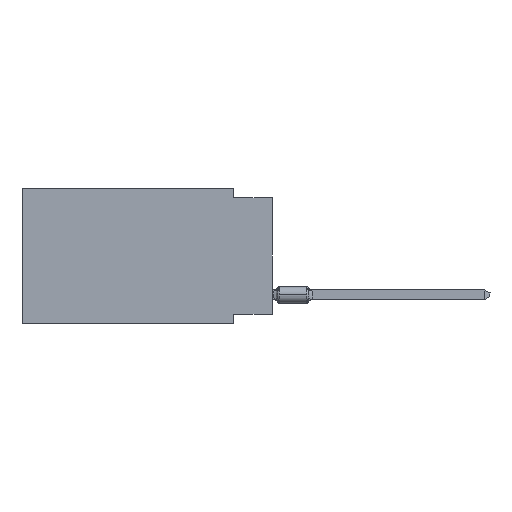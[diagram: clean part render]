
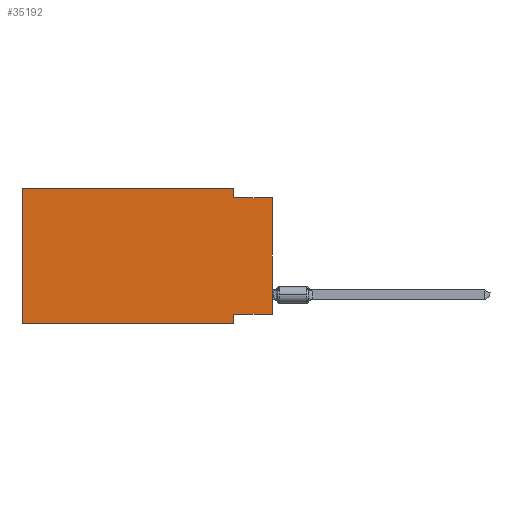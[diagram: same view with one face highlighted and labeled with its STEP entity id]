
A CAD part, left-side view. The second image highlights one B-rep face of the part: STEP entity #35192.
In plain terms, the highlighted planar face has unit normal (-1, 0, 0).
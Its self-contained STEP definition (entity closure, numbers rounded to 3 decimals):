
#883 = VECTOR ( 'NONE', #35924, 1000. ) ;
#1798 = EDGE_CURVE ( 'NONE', #45703, #31901, #57892, .T. ) ;
#2780 = VECTOR ( 'NONE', #5431, 1000. ) ;
#3551 = VECTOR ( 'NONE', #25320, 1000. ) ;
#4039 = EDGE_LOOP ( 'NONE', ( #21604, #40811, #22228, #12250, #41114, #58420, #39677, #47227 ) ) ;
#4810 = LINE ( 'NONE', #8172, #883 ) ;
#5431 = DIRECTION ( 'NONE',  ( 0., 0., 1. ) ) ;
#5694 = AXIS2_PLACEMENT_3D ( 'NONE', #21321, #26786, #53914 ) ;
#6041 = CARTESIAN_POINT ( 'NONE',  ( 0., 0., -0.635 ) ) ;
#6371 = DIRECTION ( 'NONE',  ( 0., 0., -1. ) ) ;
#7266 = CARTESIAN_POINT ( 'NONE',  ( 0., 2.54, -8.89 ) ) ;
#7728 = VECTOR ( 'NONE', #34967, 1000. ) ;
#7740 = VECTOR ( 'NONE', #36163, 1000. ) ;
#8172 = CARTESIAN_POINT ( 'NONE',  ( 0., 16.383, 0. ) ) ;
#9313 = CARTESIAN_POINT ( 'NONE',  ( 0., 2.54, -8.89 ) ) ;
#10871 = EDGE_CURVE ( 'NONE', #17451, #39127, #16458, .T. ) ;
#12250 = ORIENTED_EDGE ( 'NONE', *, *, #37661, .F. ) ;
#13617 = VECTOR ( 'NONE', #6371, 1000. ) ;
#15258 = CARTESIAN_POINT ( 'NONE',  ( 0., 16.383, 0. ) ) ;
#16373 = LINE ( 'NONE', #39853, #7728 ) ;
#16458 = LINE ( 'NONE', #15258, #3551 ) ;
#17451 = VERTEX_POINT ( 'NONE', #21964 ) ;
#17556 = CARTESIAN_POINT ( 'NONE',  ( 0., 0., -8.255 ) ) ;
#21321 = CARTESIAN_POINT ( 'NONE',  ( 0., 16.383, 0. ) ) ;
#21604 = ORIENTED_EDGE ( 'NONE', *, *, #59350, .T. ) ;
#21964 = CARTESIAN_POINT ( 'NONE',  ( 0., 16.383, -8.89 ) ) ;
#22228 = ORIENTED_EDGE ( 'NONE', *, *, #31782, .F. ) ;
#22732 = CARTESIAN_POINT ( 'NONE',  ( 0., 16.383, -8.89 ) ) ;
#25320 = DIRECTION ( 'NONE',  ( 0., 0., 1. ) ) ;
#26594 = EDGE_CURVE ( 'NONE', #46502, #45478, #47813, .T. ) ;
#26786 = DIRECTION ( 'NONE',  ( 1., 0., 0. ) ) ;
#27468 = CARTESIAN_POINT ( 'NONE',  ( 0., 2.54, -0.635 ) ) ;
#28627 = LINE ( 'NONE', #47212, #2780 ) ;
#31782 = EDGE_CURVE ( 'NONE', #58960, #46502, #16373, .T. ) ;
#31901 = VERTEX_POINT ( 'NONE', #9313 ) ;
#33528 = CARTESIAN_POINT ( 'NONE',  ( 0., 16.383, 0. ) ) ;
#34967 = DIRECTION ( 'NONE',  ( 0., 0., -1. ) ) ;
#35192 = ADVANCED_FACE ( 'NONE', ( #36250 ), #36538, .F. ) ;
#35924 = DIRECTION ( 'NONE',  ( 0., -1., 0. ) ) ;
#36163 = DIRECTION ( 'NONE',  ( 0., 1., 0. ) ) ;
#36250 = FACE_OUTER_BOUND ( 'NONE', #4039, .T. ) ;
#36538 = PLANE ( 'NONE',  #5694 ) ;
#37661 = EDGE_CURVE ( 'NONE', #39127, #58960, #4810, .T. ) ;
#39127 = VERTEX_POINT ( 'NONE', #33528 ) ;
#39677 = ORIENTED_EDGE ( 'NONE', *, *, #1798, .F. ) ;
#39853 = CARTESIAN_POINT ( 'NONE',  ( 0., 2.54, 0. ) ) ;
#40726 = LINE ( 'NONE', #17556, #7740 ) ;
#40811 = ORIENTED_EDGE ( 'NONE', *, *, #26594, .F. ) ;
#41114 = ORIENTED_EDGE ( 'NONE', *, *, #10871, .F. ) ;
#41612 = LINE ( 'NONE', #22732, #55671 ) ;
#42900 = CARTESIAN_POINT ( 'NONE',  ( 0., 0., -0.635 ) ) ;
#43234 = EDGE_CURVE ( 'NONE', #50061, #45703, #40726, .T. ) ;
#45478 = VERTEX_POINT ( 'NONE', #42900 ) ;
#45703 = VERTEX_POINT ( 'NONE', #50779 ) ;
#46502 = VERTEX_POINT ( 'NONE', #27468 ) ;
#47069 = EDGE_CURVE ( 'NONE', #17451, #31901, #41612, .T. ) ;
#47212 = CARTESIAN_POINT ( 'NONE',  ( 0., 0., 0. ) ) ;
#47227 = ORIENTED_EDGE ( 'NONE', *, *, #43234, .F. ) ;
#47813 = LINE ( 'NONE', #6041, #60154 ) ;
#50061 = VERTEX_POINT ( 'NONE', #51003 ) ;
#50779 = CARTESIAN_POINT ( 'NONE',  ( 0., 2.54, -8.255 ) ) ;
#51003 = CARTESIAN_POINT ( 'NONE',  ( 0., 0., -8.255 ) ) ;
#53914 = DIRECTION ( 'NONE',  ( 0., 0., -1. ) ) ;
#54400 = DIRECTION ( 'NONE',  ( 0., -1., 0. ) ) ;
#55671 = VECTOR ( 'NONE', #55914, 1000. ) ;
#55914 = DIRECTION ( 'NONE',  ( 0., -1., 0. ) ) ;
#57892 = LINE ( 'NONE', #7266, #13617 ) ;
#57927 = CARTESIAN_POINT ( 'NONE',  ( 0., 2.54, 0. ) ) ;
#58420 = ORIENTED_EDGE ( 'NONE', *, *, #47069, .T. ) ;
#58960 = VERTEX_POINT ( 'NONE', #57927 ) ;
#59350 = EDGE_CURVE ( 'NONE', #50061, #45478, #28627, .T. ) ;
#60154 = VECTOR ( 'NONE', #54400, 1000. ) ;
